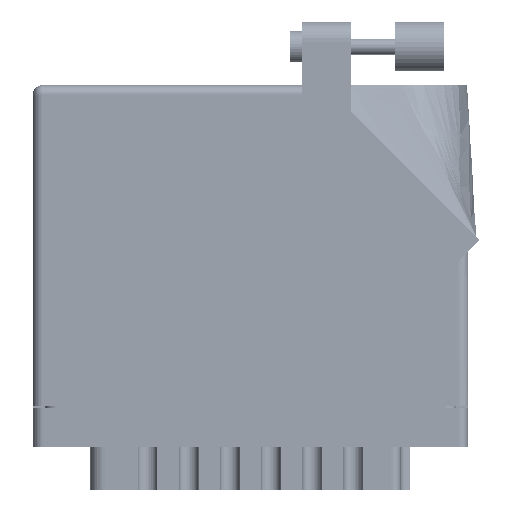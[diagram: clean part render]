
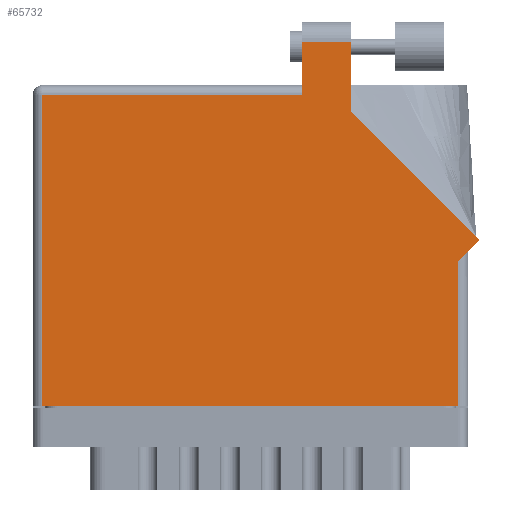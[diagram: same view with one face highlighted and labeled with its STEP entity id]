
A CAD part, front view. The second image highlights one B-rep face of the part: STEP entity #65732.
In plain terms, the highlighted face is planar.
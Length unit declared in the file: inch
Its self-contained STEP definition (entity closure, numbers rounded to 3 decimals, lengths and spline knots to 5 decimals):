
#1342 = VERTEX_POINT ( 'NONE', #42433 ) ;
#2645 = VECTOR ( 'NONE', #21224, 39.37008 ) ;
#6792 = CARTESIAN_POINT ( 'NONE',  ( 1.705, 1.968, 0. ) ) ;
#7105 = VECTOR ( 'NONE', #50616, 39.37008 ) ;
#8076 = DIRECTION ( 'NONE',  ( -1., 0., 0. ) ) ;
#8227 = LINE ( 'NONE', #93769, #7105 ) ;
#12264 = ORIENTED_EDGE ( 'NONE', *, *, #96162, .T. ) ;
#14699 = CARTESIAN_POINT ( 'NONE',  ( 2.82571, 1.05071, 0. ) ) ;
#16722 = VERTEX_POINT ( 'NONE', #80111 ) ;
#17153 = CARTESIAN_POINT ( 'NONE',  ( 1.705, 2.305, 0. ) ) ;
#17630 = CARTESIAN_POINT ( 'NONE',  ( 0.062, 1.968, 0. ) ) ;
#18531 = VECTOR ( 'NONE', #61904, 39.37008 ) ;
#20868 = LINE ( 'NONE', #54063, #18531 ) ;
#21224 = DIRECTION ( 'NONE',  ( -0.707, 0.707, 0. ) ) ;
#22442 = LINE ( 'NONE', #14699, #2645 ) ;
#22510 = LINE ( 'NONE', #17153, #38741 ) ;
#25492 = DIRECTION ( 'NONE',  ( 0., 1., 0. ) ) ;
#27444 = EDGE_CURVE ( 'NONE', #42382, #52181, #51987, .T. ) ;
#27918 = VECTOR ( 'NONE', #49587, 39.37008 ) ;
#29563 = CARTESIAN_POINT ( 'NONE',  ( 0., 2.03, 0. ) ) ;
#31939 = VERTEX_POINT ( 'NONE', #37749 ) ;
#31999 = EDGE_CURVE ( 'NONE', #61483, #63949, #20868, .T. ) ;
#36436 = PLANE ( 'NONE',  #64192 ) ;
#36483 = DIRECTION ( 'NONE',  ( 0.707, 0.707, 0. ) ) ;
#36897 = VERTEX_POINT ( 'NONE', #52189 ) ;
#37474 = VECTOR ( 'NONE', #25492, 39.37008 ) ;
#37749 = CARTESIAN_POINT ( 'NONE',  ( 2.012, 2.305, 0. ) ) ;
#38672 = FACE_OUTER_BOUND ( 'NONE', #90146, .T. ) ;
#38741 = VECTOR ( 'NONE', #84026, 39.37008 ) ;
#38827 = ORIENTED_EDGE ( 'NONE', *, *, #71696, .T. ) ;
#39797 = CARTESIAN_POINT ( 'NONE',  ( 2.693, 0.98, 0. ) ) ;
#39931 = ORIENTED_EDGE ( 'NONE', *, *, #31999, .T. ) ;
#41133 = EDGE_CURVE ( 'NONE', #63949, #16722, #8227, .T. ) ;
#42382 = VERTEX_POINT ( 'NONE', #45628 ) ;
#42433 = CARTESIAN_POINT ( 'NONE',  ( 2.012, 1.86442, 0. ) ) ;
#44426 = VECTOR ( 'NONE', #92733, 39.37008 ) ;
#44496 = LINE ( 'NONE', #54511, #37474 ) ;
#44543 = DIRECTION ( 'NONE',  ( 0., 0., -1. ) ) ;
#45270 = DIRECTION ( 'NONE',  ( -1., 0., 0. ) ) ;
#45628 = CARTESIAN_POINT ( 'NONE',  ( 2.693, 0.918, 0. ) ) ;
#46384 = VERTEX_POINT ( 'NONE', #6792 ) ;
#46434 = CARTESIAN_POINT ( 'NONE',  ( 2.755, 0.98, 0. ) ) ;
#49587 = DIRECTION ( 'NONE',  ( 0., -1., 0. ) ) ;
#50616 = DIRECTION ( 'NONE',  ( 1., 0., 0. ) ) ;
#51233 = ORIENTED_EDGE ( 'NONE', *, *, #41133, .T. ) ;
#51987 = LINE ( 'NONE', #46434, #59036 ) ;
#52181 = VERTEX_POINT ( 'NONE', #63515 ) ;
#52189 = CARTESIAN_POINT ( 'NONE',  ( 1.705, 2.305, 0. ) ) ;
#54063 = CARTESIAN_POINT ( 'NONE',  ( 0.062, 0., 0. ) ) ;
#54511 = CARTESIAN_POINT ( 'NONE',  ( 2.012, 1.86442, 0. ) ) ;
#55862 = EDGE_CURVE ( 'NONE', #36897, #46384, #60554, .T. ) ;
#58326 = ORIENTED_EDGE ( 'NONE', *, *, #89760, .T. ) ;
#59036 = VECTOR ( 'NONE', #36483, 39.37008 ) ;
#59919 = EDGE_CURVE ( 'NONE', #52181, #1342, #22442, .T. ) ;
#60554 = LINE ( 'NONE', #94348, #27918 ) ;
#61133 = LINE ( 'NONE', #67810, #84524 ) ;
#61483 = VERTEX_POINT ( 'NONE', #17630 ) ;
#61904 = DIRECTION ( 'NONE',  ( 0., -1., 0. ) ) ;
#63515 = CARTESIAN_POINT ( 'NONE',  ( 2.82571, 1.05071, 0. ) ) ;
#63949 = VERTEX_POINT ( 'NONE', #95231 ) ;
#64192 = AXIS2_PLACEMENT_3D ( 'NONE', #29563, #44543, #8076 ) ;
#65732 = ADVANCED_FACE ( 'NONE', ( #38672 ), #36436, .F. ) ;
#67810 = CARTESIAN_POINT ( 'NONE',  ( 0., 1.968, 0. ) ) ;
#70825 = EDGE_CURVE ( 'NONE', #46384, #61483, #61133, .T. ) ;
#71696 = EDGE_CURVE ( 'NONE', #31939, #36897, #22510, .T. ) ;
#74627 = ORIENTED_EDGE ( 'NONE', *, *, #27444, .T. ) ;
#77972 = ORIENTED_EDGE ( 'NONE', *, *, #55862, .T. ) ;
#80111 = CARTESIAN_POINT ( 'NONE',  ( 2.693, 0., 0. ) ) ;
#84026 = DIRECTION ( 'NONE',  ( -1., 0., 0. ) ) ;
#84524 = VECTOR ( 'NONE', #45270, 39.37008 ) ;
#88369 = ORIENTED_EDGE ( 'NONE', *, *, #59919, .T. ) ;
#89760 = EDGE_CURVE ( 'NONE', #16722, #42382, #91234, .T. ) ;
#90146 = EDGE_LOOP ( 'NONE', ( #12264, #38827, #77972, #91240, #39931, #51233, #58326, #74627, #88369 ) ) ;
#91234 = LINE ( 'NONE', #39797, #44426 ) ;
#91240 = ORIENTED_EDGE ( 'NONE', *, *, #70825, .T. ) ;
#92733 = DIRECTION ( 'NONE',  ( 0., 1., 0. ) ) ;
#93769 = CARTESIAN_POINT ( 'NONE',  ( 0., 0., 0. ) ) ;
#94348 = CARTESIAN_POINT ( 'NONE',  ( 1.705, 2.03, 0. ) ) ;
#95231 = CARTESIAN_POINT ( 'NONE',  ( 0.062, 0., 0. ) ) ;
#96162 = EDGE_CURVE ( 'NONE', #1342, #31939, #44496, .T. ) ;
